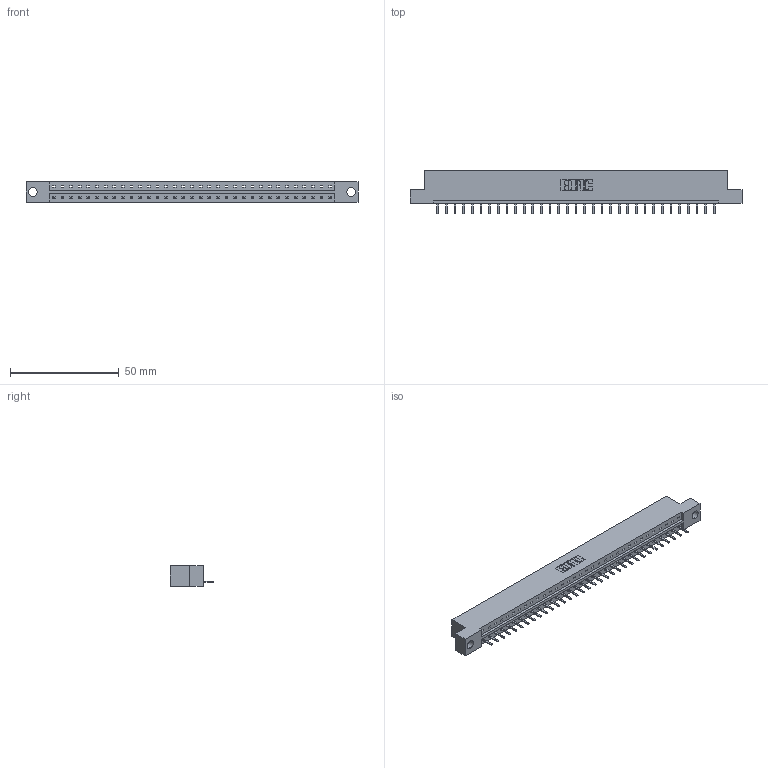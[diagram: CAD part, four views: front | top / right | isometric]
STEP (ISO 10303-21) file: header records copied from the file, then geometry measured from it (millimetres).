
FILE_DESCRIPTION (( 'STEP AP203' ), '1' );
FILE_NAME ('833-033-520-104.STEP', '2020-06-02T19:46:17', ( '' ), ( '' ), 'SwSTEP 2.0', 'SolidWorks 2020', '' );
FILE_SCHEMA (( 'CONFIG_CONTROL_DESIGN' ));
Length unit declared in the file: inch
Products named in the file (3): 833 Part_Flush - .156 Dia - TH; 833-033-520-104; 345-292-001_345-293-120
Assembly tree (34 placements, depth 2):
  833-033-520-104
    833 Part_Flush - .156 Dia - TH
    345-292-001_345-293-120  x33
Bounding box: 152.3 x 20.02 x 9.4 mm (x, y, z)
Volume: 15065.3 mm3; surface area: 15703.9 mm2
Topology: 34 solids, 34 shells, 2160 faces, 6383 edges, 4166 vertices
Faces by surface type: plane 1522, cylinder 638
Entity records: 21455 total; most frequent: CARTESIAN_POINT 3721, ORIENTED_EDGE 3678, DIRECTION 3145, EDGE_CURVE 1839, LINE 1707, VECTOR 1707, VERTEX_POINT 1222, AXIS2_PLACEMENT_3D 719
